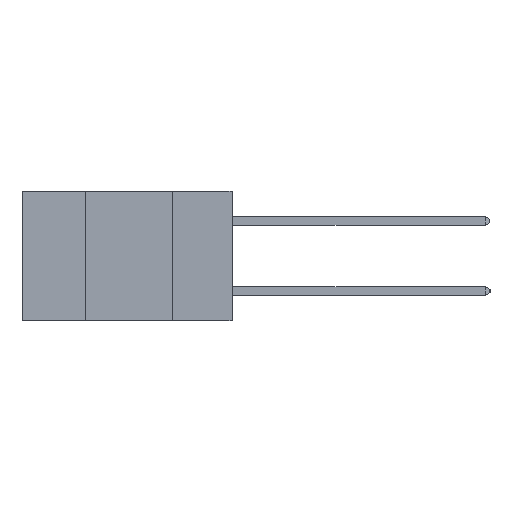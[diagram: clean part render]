
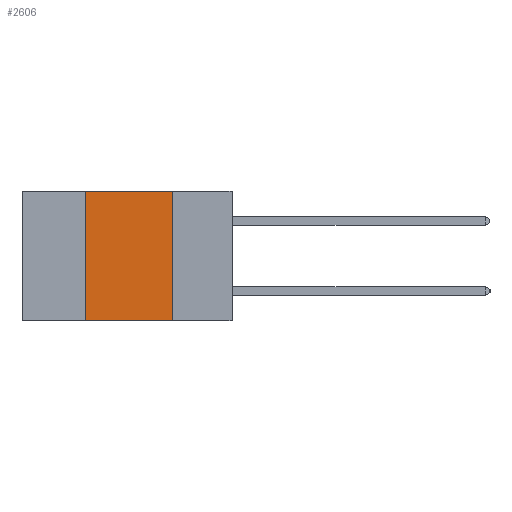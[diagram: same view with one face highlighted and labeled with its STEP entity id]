
A CAD part, left-side view. The second image highlights one B-rep face of the part: STEP entity #2606.
In plain terms, the highlighted planar face has unit normal (-1, 0, 0).
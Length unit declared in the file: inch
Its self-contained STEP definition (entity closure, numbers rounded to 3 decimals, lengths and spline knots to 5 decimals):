
#1292 = DIRECTION ( 'NONE',  ( 0., 0., 1. ) ) ;
#2163 = ORIENTED_EDGE ( 'NONE', *, *, #15260, .F. ) ;
#2606 = ADVANCED_FACE ( 'NONE', ( #16996 ), #7183, .F. ) ;
#3038 = DIRECTION ( 'NONE',  ( 0., -1., 0. ) ) ;
#3756 = VECTOR ( 'NONE', #3038, 39.37008 ) ;
#3775 = LINE ( 'NONE', #4130, #21003 ) ;
#3921 = DIRECTION ( 'NONE',  ( 1., 0., 0. ) ) ;
#4130 = CARTESIAN_POINT ( 'NONE',  ( 0., 0.6, 0. ) ) ;
#4208 = VERTEX_POINT ( 'NONE', #15585 ) ;
#4705 = CARTESIAN_POINT ( 'NONE',  ( 0., 0.6, -0.37 ) ) ;
#4802 = DIRECTION ( 'NONE',  ( 0., 0., -1. ) ) ;
#5470 = CARTESIAN_POINT ( 'NONE',  ( 0., 0.42, -0.37 ) ) ;
#5856 = VECTOR ( 'NONE', #1292, 39.37008 ) ;
#7183 = PLANE ( 'NONE',  #21690 ) ;
#7406 = VERTEX_POINT ( 'NONE', #9516 ) ;
#7503 = EDGE_CURVE ( 'NONE', #16959, #7406, #12711, .T. ) ;
#8158 = CARTESIAN_POINT ( 'NONE',  ( 0., 0.6, 0. ) ) ;
#9285 = EDGE_LOOP ( 'NONE', ( #13242, #21227, #2163, #18636 ) ) ;
#9516 = CARTESIAN_POINT ( 'NONE',  ( 0., 0.17, -0.37 ) ) ;
#12711 = LINE ( 'NONE', #4705, #3756 ) ;
#13150 = CARTESIAN_POINT ( 'NONE',  ( 0., 0.17, 0. ) ) ;
#13242 = ORIENTED_EDGE ( 'NONE', *, *, #15979, .F. ) ;
#14145 = LINE ( 'NONE', #19685, #5856 ) ;
#14342 = VERTEX_POINT ( 'NONE', #20288 ) ;
#15260 = EDGE_CURVE ( 'NONE', #16959, #14342, #14145, .T. ) ;
#15585 = CARTESIAN_POINT ( 'NONE',  ( 0., 0.17, 0. ) ) ;
#15979 = EDGE_CURVE ( 'NONE', #4208, #7406, #17212, .T. ) ;
#16959 = VERTEX_POINT ( 'NONE', #5470 ) ;
#16996 = FACE_OUTER_BOUND ( 'NONE', #9285, .T. ) ;
#17212 = LINE ( 'NONE', #13150, #21122 ) ;
#17652 = DIRECTION ( 'NONE',  ( 0., 0., -1. ) ) ;
#18636 = ORIENTED_EDGE ( 'NONE', *, *, #7503, .T. ) ;
#19685 = CARTESIAN_POINT ( 'NONE',  ( 0., 0.42, 0. ) ) ;
#20288 = CARTESIAN_POINT ( 'NONE',  ( 0., 0.42, 0. ) ) ;
#20580 = EDGE_CURVE ( 'NONE', #14342, #4208, #3775, .T. ) ;
#20808 = DIRECTION ( 'NONE',  ( 0., -1., 0. ) ) ;
#21003 = VECTOR ( 'NONE', #20808, 39.37008 ) ;
#21122 = VECTOR ( 'NONE', #4802, 39.37008 ) ;
#21227 = ORIENTED_EDGE ( 'NONE', *, *, #20580, .F. ) ;
#21690 = AXIS2_PLACEMENT_3D ( 'NONE', #8158, #3921, #17652 ) ;
